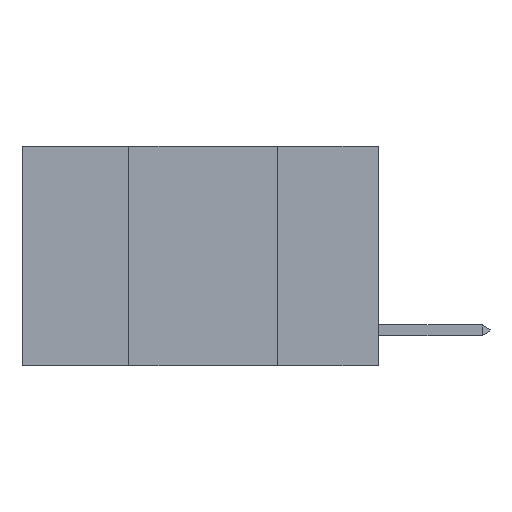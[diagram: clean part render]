
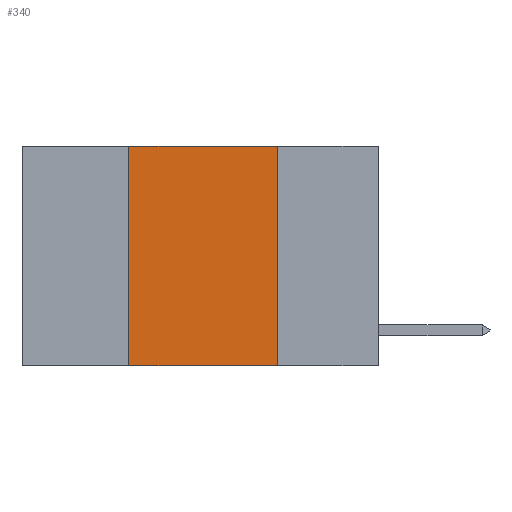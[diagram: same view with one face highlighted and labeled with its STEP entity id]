
A CAD part, left-side view. The second image highlights one B-rep face of the part: STEP entity #340.
In plain terms, the highlighted planar face has unit normal (-1, 0, 0).
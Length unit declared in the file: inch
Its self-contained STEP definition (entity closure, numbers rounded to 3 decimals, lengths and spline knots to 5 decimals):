
#228 = VECTOR ( 'NONE', #7282, 39.37008 ) ;
#340 = ADVANCED_FACE ( 'NONE', ( #5825 ), #8449, .F. ) ;
#555 = EDGE_CURVE ( 'NONE', #8814, #2885, #688, .T. ) ;
#688 = LINE ( 'NONE', #1484, #228 ) ;
#912 = VECTOR ( 'NONE', #6584, 39.37008 ) ;
#1454 = EDGE_CURVE ( 'NONE', #5188, #2480, #3125, .T. ) ;
#1484 = CARTESIAN_POINT ( 'NONE',  ( 0., 0.6, 0. ) ) ;
#1809 = VECTOR ( 'NONE', #8520, 39.37008 ) ;
#2403 = CARTESIAN_POINT ( 'NONE',  ( 0., 0.17, 0. ) ) ;
#2453 = DIRECTION ( 'NONE',  ( 1., 0., 0. ) ) ;
#2480 = VERTEX_POINT ( 'NONE', #9118 ) ;
#2641 = EDGE_CURVE ( 'NONE', #5188, #8814, #4601, .T. ) ;
#2885 = VERTEX_POINT ( 'NONE', #10558 ) ;
#3125 = LINE ( 'NONE', #6431, #912 ) ;
#3172 = LINE ( 'NONE', #2403, #8624 ) ;
#3462 = CARTESIAN_POINT ( 'NONE',  ( 0., 0.42, -0.37 ) ) ;
#4201 = CARTESIAN_POINT ( 'NONE',  ( 0., 0.42, 0. ) ) ;
#4432 = CARTESIAN_POINT ( 'NONE',  ( 0., 0.42, 0. ) ) ;
#4601 = LINE ( 'NONE', #4432, #1809 ) ;
#5078 = DIRECTION ( 'NONE',  ( 0., 0., -1. ) ) ;
#5188 = VERTEX_POINT ( 'NONE', #3462 ) ;
#5825 = FACE_OUTER_BOUND ( 'NONE', #9871, .T. ) ;
#5898 = ORIENTED_EDGE ( 'NONE', *, *, #555, .F. ) ;
#6431 = CARTESIAN_POINT ( 'NONE',  ( 0., 0.6, -0.37 ) ) ;
#6584 = DIRECTION ( 'NONE',  ( 0., -1., 0. ) ) ;
#7204 = DIRECTION ( 'NONE',  ( 0., 0., -1. ) ) ;
#7282 = DIRECTION ( 'NONE',  ( 0., -1., 0. ) ) ;
#7377 = ORIENTED_EDGE ( 'NONE', *, *, #1454, .T. ) ;
#7576 = CARTESIAN_POINT ( 'NONE',  ( 0., 0.6, 0. ) ) ;
#7960 = ORIENTED_EDGE ( 'NONE', *, *, #10702, .F. ) ;
#8449 = PLANE ( 'NONE',  #9401 ) ;
#8520 = DIRECTION ( 'NONE',  ( 0., 0., 1. ) ) ;
#8624 = VECTOR ( 'NONE', #7204, 39.37008 ) ;
#8814 = VERTEX_POINT ( 'NONE', #4201 ) ;
#8958 = ORIENTED_EDGE ( 'NONE', *, *, #2641, .F. ) ;
#9118 = CARTESIAN_POINT ( 'NONE',  ( 0., 0.17, -0.37 ) ) ;
#9401 = AXIS2_PLACEMENT_3D ( 'NONE', #7576, #2453, #5078 ) ;
#9871 = EDGE_LOOP ( 'NONE', ( #7960, #5898, #8958, #7377 ) ) ;
#10558 = CARTESIAN_POINT ( 'NONE',  ( 0., 0.17, 0. ) ) ;
#10702 = EDGE_CURVE ( 'NONE', #2885, #2480, #3172, .T. ) ;
